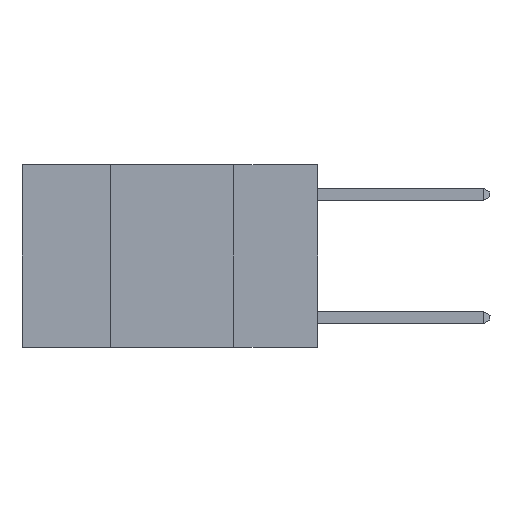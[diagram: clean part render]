
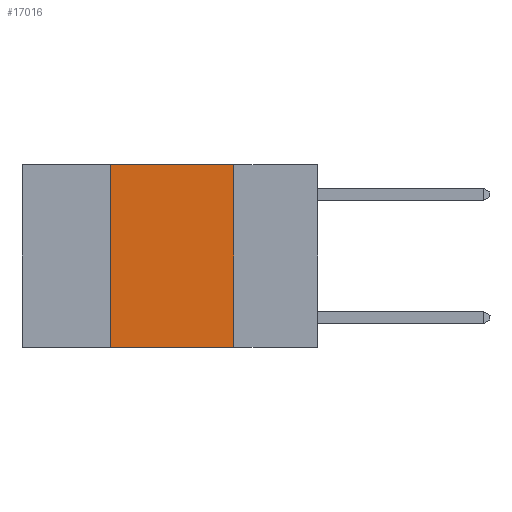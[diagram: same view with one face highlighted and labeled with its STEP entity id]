
A CAD part, left-side view. The second image highlights one B-rep face of the part: STEP entity #17016.
In plain terms, the highlighted planar face has unit normal (-1, 0, 0).
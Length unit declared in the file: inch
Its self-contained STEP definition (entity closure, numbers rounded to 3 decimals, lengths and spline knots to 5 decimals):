
#364 = DIRECTION ( 'NONE',  ( 0., -1., 0. ) ) ;
#779 = DIRECTION ( 'NONE',  ( 1., 0., 0. ) ) ;
#1001 = DIRECTION ( 'NONE',  ( 0., -1., 0. ) ) ;
#1751 = LINE ( 'NONE', #9333, #15944 ) ;
#2079 = FACE_OUTER_BOUND ( 'NONE', #11200, .T. ) ;
#2134 = VECTOR ( 'NONE', #1001, 39.37008 ) ;
#3657 = LINE ( 'NONE', #15513, #14723 ) ;
#3735 = CARTESIAN_POINT ( 'NONE',  ( 0., 0.42, -0.37 ) ) ;
#4887 = ORIENTED_EDGE ( 'NONE', *, *, #8173, .F. ) ;
#5442 = LINE ( 'NONE', #10776, #2134 ) ;
#7344 = DIRECTION ( 'NONE',  ( 0., 0., -1. ) ) ;
#7791 = CARTESIAN_POINT ( 'NONE',  ( 0., 0.6, 0. ) ) ;
#8173 = EDGE_CURVE ( 'NONE', #17450, #14076, #3657, .T. ) ;
#8528 = EDGE_CURVE ( 'NONE', #13039, #14076, #5442, .T. ) ;
#8638 = ORIENTED_EDGE ( 'NONE', *, *, #16827, .F. ) ;
#8686 = CARTESIAN_POINT ( 'NONE',  ( 0., 0.17, 0. ) ) ;
#9305 = LINE ( 'NONE', #10142, #12971 ) ;
#9333 = CARTESIAN_POINT ( 'NONE',  ( 0., 0.42, 0. ) ) ;
#9530 = CARTESIAN_POINT ( 'NONE',  ( 0., 0.42, 0. ) ) ;
#10142 = CARTESIAN_POINT ( 'NONE',  ( 0., 0.6, 0. ) ) ;
#10453 = CARTESIAN_POINT ( 'NONE',  ( 0., 0.17, -0.37 ) ) ;
#10559 = DIRECTION ( 'NONE',  ( 0., 0., -1. ) ) ;
#10776 = CARTESIAN_POINT ( 'NONE',  ( 0., 0.6, -0.37 ) ) ;
#11200 = EDGE_LOOP ( 'NONE', ( #4887, #8638, #12275, #15821 ) ) ;
#11258 = VERTEX_POINT ( 'NONE', #9530 ) ;
#12275 = ORIENTED_EDGE ( 'NONE', *, *, #14927, .F. ) ;
#12971 = VECTOR ( 'NONE', #364, 39.37008 ) ;
#13039 = VERTEX_POINT ( 'NONE', #3735 ) ;
#14076 = VERTEX_POINT ( 'NONE', #10453 ) ;
#14723 = VECTOR ( 'NONE', #7344, 39.37008 ) ;
#14833 = DIRECTION ( 'NONE',  ( 0., 0., 1. ) ) ;
#14872 = AXIS2_PLACEMENT_3D ( 'NONE', #7791, #779, #10559 ) ;
#14927 = EDGE_CURVE ( 'NONE', #13039, #11258, #1751, .T. ) ;
#15513 = CARTESIAN_POINT ( 'NONE',  ( 0., 0.17, 0. ) ) ;
#15821 = ORIENTED_EDGE ( 'NONE', *, *, #8528, .T. ) ;
#15944 = VECTOR ( 'NONE', #14833, 39.37008 ) ;
#16827 = EDGE_CURVE ( 'NONE', #11258, #17450, #9305, .T. ) ;
#17016 = ADVANCED_FACE ( 'NONE', ( #2079 ), #17210, .F. ) ;
#17210 = PLANE ( 'NONE',  #14872 ) ;
#17450 = VERTEX_POINT ( 'NONE', #8686 ) ;
